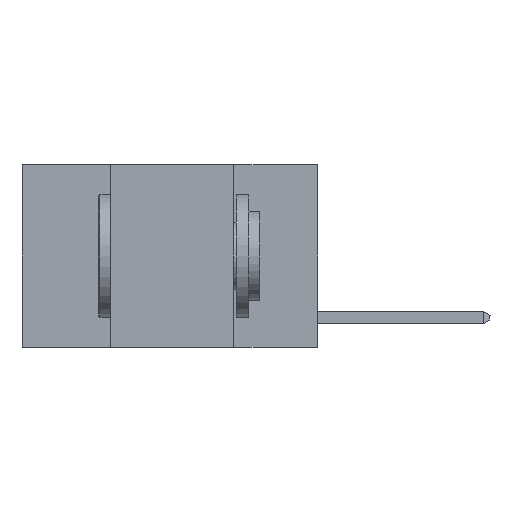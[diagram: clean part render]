
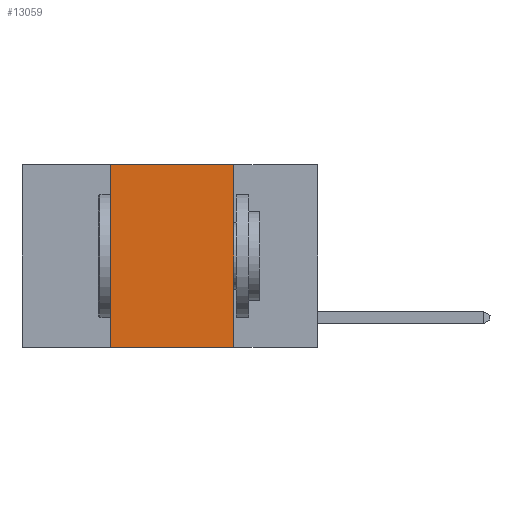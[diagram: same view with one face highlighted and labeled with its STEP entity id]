
A CAD part, left-side view. The second image highlights one B-rep face of the part: STEP entity #13059.
In plain terms, the highlighted planar face has unit normal (-1, 0, 0).
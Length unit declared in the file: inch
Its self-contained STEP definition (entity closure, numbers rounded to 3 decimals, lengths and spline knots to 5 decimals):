
#493 = ORIENTED_EDGE ( 'NONE', *, *, #3093, .F. ) ;
#1031 = VERTEX_POINT ( 'NONE', #9438 ) ;
#1118 = EDGE_CURVE ( 'NONE', #1031, #10624, #13049, .T. ) ;
#1233 = EDGE_CURVE ( 'NONE', #1878, #7088, #12948, .T. ) ;
#1878 = VERTEX_POINT ( 'NONE', #7808 ) ;
#2528 = ORIENTED_EDGE ( 'NONE', *, *, #1118, .F. ) ;
#3093 = EDGE_CURVE ( 'NONE', #10624, #7088, #14561, .T. ) ;
#3360 = CARTESIAN_POINT ( 'NONE',  ( 0., 0.42, 0. ) ) ;
#3986 = CARTESIAN_POINT ( 'NONE',  ( 0., 0.6, -0.37 ) ) ;
#4096 = VECTOR ( 'NONE', #18163, 39.37008 ) ;
#4436 = FACE_OUTER_BOUND ( 'NONE', #16908, .T. ) ;
#4925 = CARTESIAN_POINT ( 'NONE',  ( 0., 0.17, -0.37 ) ) ;
#5812 = PLANE ( 'NONE',  #18366 ) ;
#7088 = VERTEX_POINT ( 'NONE', #4925 ) ;
#7808 = CARTESIAN_POINT ( 'NONE',  ( 0., 0.42, -0.37 ) ) ;
#9438 = CARTESIAN_POINT ( 'NONE',  ( 0., 0.42, 0. ) ) ;
#10569 = LINE ( 'NONE', #3360, #4096 ) ;
#10624 = VERTEX_POINT ( 'NONE', #18403 ) ;
#11631 = DIRECTION ( 'NONE',  ( 0., 0., -1. ) ) ;
#12442 = ORIENTED_EDGE ( 'NONE', *, *, #12716, .F. ) ;
#12716 = EDGE_CURVE ( 'NONE', #1878, #1031, #10569, .T. ) ;
#12948 = LINE ( 'NONE', #3986, #18316 ) ;
#13001 = DIRECTION ( 'NONE',  ( 1., 0., 0. ) ) ;
#13049 = LINE ( 'NONE', #15910, #16117 ) ;
#13059 = ADVANCED_FACE ( 'NONE', ( #4436 ), #5812, .F. ) ;
#14332 = ORIENTED_EDGE ( 'NONE', *, *, #1233, .T. ) ;
#14471 = CARTESIAN_POINT ( 'NONE',  ( 0., 0.17, 0. ) ) ;
#14561 = LINE ( 'NONE', #14471, #16925 ) ;
#15798 = DIRECTION ( 'NONE',  ( 0., -1., 0. ) ) ;
#15910 = CARTESIAN_POINT ( 'NONE',  ( 0., 0.6, 0. ) ) ;
#16019 = DIRECTION ( 'NONE',  ( 0., -1., 0. ) ) ;
#16048 = DIRECTION ( 'NONE',  ( 0., 0., -1. ) ) ;
#16117 = VECTOR ( 'NONE', #15798, 39.37008 ) ;
#16908 = EDGE_LOOP ( 'NONE', ( #493, #2528, #12442, #14332 ) ) ;
#16925 = VECTOR ( 'NONE', #16048, 39.37008 ) ;
#18163 = DIRECTION ( 'NONE',  ( 0., 0., 1. ) ) ;
#18316 = VECTOR ( 'NONE', #16019, 39.37008 ) ;
#18366 = AXIS2_PLACEMENT_3D ( 'NONE', #19128, #13001, #11631 ) ;
#18403 = CARTESIAN_POINT ( 'NONE',  ( 0., 0.17, 0. ) ) ;
#19128 = CARTESIAN_POINT ( 'NONE',  ( 0., 0.6, 0. ) ) ;
